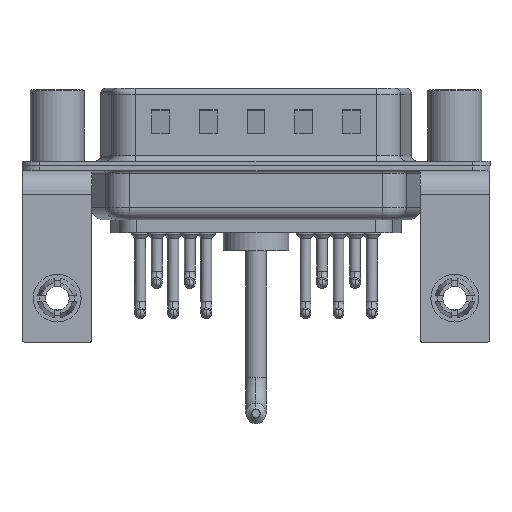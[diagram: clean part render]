
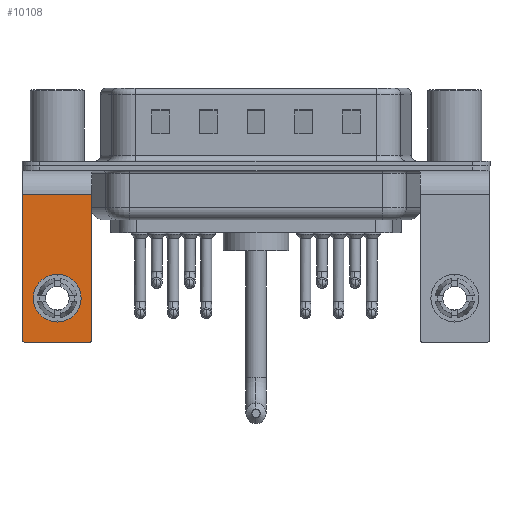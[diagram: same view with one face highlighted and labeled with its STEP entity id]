
A CAD part, front view. The second image highlights one B-rep face of the part: STEP entity #10108.
In plain terms, the highlighted planar face has unit normal (0, -1, 0).
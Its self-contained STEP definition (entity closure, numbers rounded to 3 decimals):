
#664 = FACE_OUTER_BOUND ( 'NONE', #3133, .T. ) ;
#864 = CARTESIAN_POINT ( 'NONE',  ( -2.9, -6.25, -14.55 ) ) ;
#1500 = DIRECTION ( 'NONE',  ( 0., -1., 0. ) ) ;
#2173 = EDGE_CURVE ( 'NONE', #26260, #19344, #23846, .T. ) ;
#2437 = EDGE_CURVE ( 'NONE', #26260, #17035, #16105, .T. ) ;
#2496 = DIRECTION ( 'NONE',  ( 0., 0., 1. ) ) ;
#2697 = ORIENTED_EDGE ( 'NONE', *, *, #26396, .T. ) ;
#3133 = EDGE_LOOP ( 'NONE', ( #4613, #18357, #24752, #11651, #14669, #20289 ) ) ;
#3871 = VECTOR ( 'NONE', #6883, 1000. ) ;
#4408 = CARTESIAN_POINT ( 'NONE',  ( -2.9, -6.25, -2.4 ) ) ;
#4480 = LINE ( 'NONE', #15205, #3871 ) ;
#4613 = ORIENTED_EDGE ( 'NONE', *, *, #4652, .T. ) ;
#4652 = EDGE_CURVE ( 'NONE', #14538, #9381, #14731, .T. ) ;
#4899 = VERTEX_POINT ( 'NONE', #15395 ) ;
#5910 = DIRECTION ( 'NONE',  ( 0., 0., 1. ) ) ;
#6305 = FACE_BOUND ( 'NONE', #18484, .T. ) ;
#6883 = DIRECTION ( 'NONE',  ( 0., 0., -1. ) ) ;
#7174 = CARTESIAN_POINT ( 'NONE',  ( 0., -6.25, -11.07 ) ) ;
#7553 = AXIS2_PLACEMENT_3D ( 'NONE', #19870, #1500, #24019 ) ;
#7928 = DIRECTION ( 'NONE',  ( 0., 1., 0. ) ) ;
#8302 = DIRECTION ( 'NONE',  ( 0., 0., -1. ) ) ;
#9381 = VERTEX_POINT ( 'NONE', #864 ) ;
#9751 = CARTESIAN_POINT ( 'NONE',  ( 2.9, -6.25, -2.4 ) ) ;
#10108 = ADVANCED_FACE ( 'NONE', ( #6305, #664 ), #12878, .F. ) ;
#10277 = ORIENTED_EDGE ( 'NONE', *, *, #23155, .T. ) ;
#11356 = EDGE_CURVE ( 'NONE', #11726, #19344, #4480, .T. ) ;
#11651 = ORIENTED_EDGE ( 'NONE', *, *, #2173, .T. ) ;
#11726 = VERTEX_POINT ( 'NONE', #25523 ) ;
#12314 = VECTOR ( 'NONE', #18245, 1000. ) ;
#12878 = PLANE ( 'NONE',  #25653 ) ;
#13350 = EDGE_CURVE ( 'NONE', #11726, #14538, #18186, .T. ) ;
#13901 = DIRECTION ( 'NONE',  ( -1., 0., 0. ) ) ;
#14409 = CARTESIAN_POINT ( 'NONE',  ( -2.65, -6.25, -14.8 ) ) ;
#14538 = VERTEX_POINT ( 'NONE', #20799 ) ;
#14624 = DIRECTION ( 'NONE',  ( 0., 1., 0. ) ) ;
#14669 = ORIENTED_EDGE ( 'NONE', *, *, #11356, .F. ) ;
#14731 = LINE ( 'NONE', #4408, #25622 ) ;
#15179 = DIRECTION ( 'NONE',  ( 0., 0., 1. ) ) ;
#15205 = CARTESIAN_POINT ( 'NONE',  ( 2.9, -6.25, -2.4 ) ) ;
#15395 = CARTESIAN_POINT ( 'NONE',  ( 0., -6.25, -9.07 ) ) ;
#15686 = CIRCLE ( 'NONE', #7553, 0.25 ) ;
#16105 = LINE ( 'NONE', #22249, #12314 ) ;
#16490 = CIRCLE ( 'NONE', #18192, 2. ) ;
#17035 = VERTEX_POINT ( 'NONE', #14409 ) ;
#17447 = CARTESIAN_POINT ( 'NONE',  ( 2.65, -6.25, -14.55 ) ) ;
#17761 = VERTEX_POINT ( 'NONE', #19454 ) ;
#18186 = LINE ( 'NONE', #9751, #22287 ) ;
#18192 = AXIS2_PLACEMENT_3D ( 'NONE', #20533, #7928, #5910 ) ;
#18245 = DIRECTION ( 'NONE',  ( -1., 0., 0. ) ) ;
#18357 = ORIENTED_EDGE ( 'NONE', *, *, #25888, .T. ) ;
#18484 = EDGE_LOOP ( 'NONE', ( #10277, #2697 ) ) ;
#19151 = AXIS2_PLACEMENT_3D ( 'NONE', #17447, #25493, #15179 ) ;
#19248 = DIRECTION ( 'NONE',  ( 0., 1., 0. ) ) ;
#19344 = VERTEX_POINT ( 'NONE', #26177 ) ;
#19454 = CARTESIAN_POINT ( 'NONE',  ( 0., -6.25, -13.07 ) ) ;
#19870 = CARTESIAN_POINT ( 'NONE',  ( -2.65, -6.25, -14.55 ) ) ;
#20289 = ORIENTED_EDGE ( 'NONE', *, *, #13350, .T. ) ;
#20469 = CARTESIAN_POINT ( 'NONE',  ( 2.65, -6.25, -14.8 ) ) ;
#20533 = CARTESIAN_POINT ( 'NONE',  ( 0., -6.25, -11.07 ) ) ;
#20658 = DIRECTION ( 'NONE',  ( 0., 0., 1. ) ) ;
#20799 = CARTESIAN_POINT ( 'NONE',  ( -2.9, -6.25, -2.4 ) ) ;
#22249 = CARTESIAN_POINT ( 'NONE',  ( 2.9, -6.25, -14.8 ) ) ;
#22287 = VECTOR ( 'NONE', #13901, 1000. ) ;
#22966 = AXIS2_PLACEMENT_3D ( 'NONE', #7174, #19248, #2496 ) ;
#23155 = EDGE_CURVE ( 'NONE', #17761, #4899, #16490, .T. ) ;
#23846 = CIRCLE ( 'NONE', #19151, 0.25 ) ;
#24019 = DIRECTION ( 'NONE',  ( 0., 0., 1. ) ) ;
#24241 = CIRCLE ( 'NONE', #22966, 2. ) ;
#24752 = ORIENTED_EDGE ( 'NONE', *, *, #2437, .F. ) ;
#25060 = CARTESIAN_POINT ( 'NONE',  ( 2.9, -6.25, -2.4 ) ) ;
#25493 = DIRECTION ( 'NONE',  ( 0., -1., 0. ) ) ;
#25523 = CARTESIAN_POINT ( 'NONE',  ( 2.9, -6.25, -2.4 ) ) ;
#25622 = VECTOR ( 'NONE', #8302, 1000. ) ;
#25653 = AXIS2_PLACEMENT_3D ( 'NONE', #25060, #14624, #20658 ) ;
#25888 = EDGE_CURVE ( 'NONE', #9381, #17035, #15686, .T. ) ;
#26177 = CARTESIAN_POINT ( 'NONE',  ( 2.9, -6.25, -14.55 ) ) ;
#26260 = VERTEX_POINT ( 'NONE', #20469 ) ;
#26396 = EDGE_CURVE ( 'NONE', #4899, #17761, #24241, .T. ) ;
